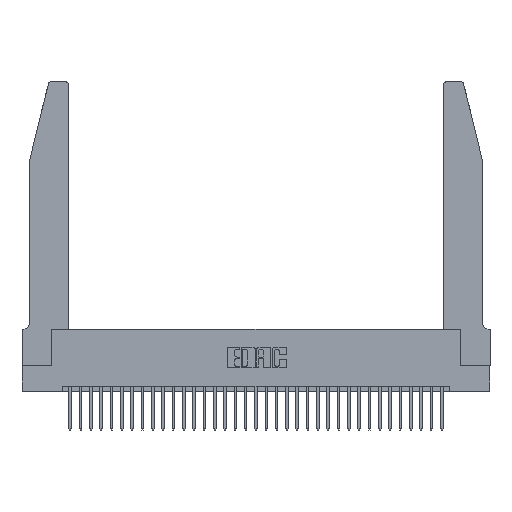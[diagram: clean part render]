
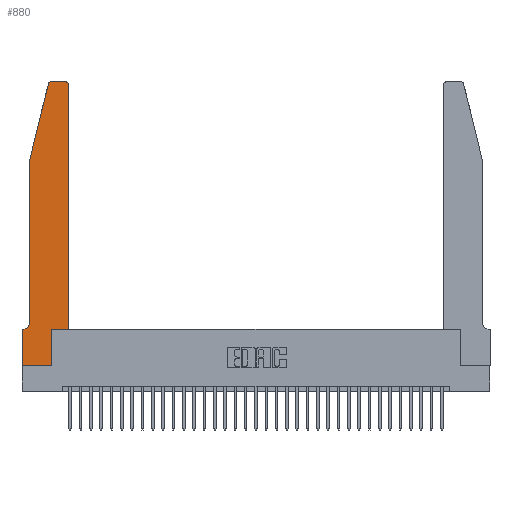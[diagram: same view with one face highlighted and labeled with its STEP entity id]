
A CAD part, top view. The second image highlights one B-rep face of the part: STEP entity #880.
In plain terms, the highlighted planar face has unit normal (0, 0, 1).
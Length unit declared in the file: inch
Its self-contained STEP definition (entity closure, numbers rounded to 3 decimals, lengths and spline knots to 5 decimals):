
#388 = CARTESIAN_POINT ( 'NONE',  ( 0.4505, 0.35, 0.37 ) ) ;
#748 = AXIS2_PLACEMENT_3D ( 'NONE', #17738, #28387, #12498 ) ;
#880 = ADVANCED_FACE ( 'NONE', ( #8861 ), #9839, .T. ) ;
#884 = EDGE_CURVE ( 'NONE', #30929, #30407, #30021, .T. ) ;
#1412 = EDGE_CURVE ( 'NONE', #30407, #5134, #1619, .T. ) ;
#1475 = ORIENTED_EDGE ( 'NONE', *, *, #4021, .T. ) ;
#1619 = CIRCLE ( 'NONE', #23368, 0.03 ) ;
#1680 = CARTESIAN_POINT ( 'NONE',  ( 0.0755, 2., 0.37 ) ) ;
#2343 = ORIENTED_EDGE ( 'NONE', *, *, #17369, .T. ) ;
#2407 = CARTESIAN_POINT ( 'NONE',  ( 0.2865, 0.35, 0.37 ) ) ;
#2535 = VERTEX_POINT ( 'NONE', #22424 ) ;
#2553 = VERTEX_POINT ( 'NONE', #30493 ) ;
#2742 = CARTESIAN_POINT ( 'NONE',  ( 0., 0., 0.37 ) ) ;
#2845 = DIRECTION ( 'NONE',  ( -1., 0., 0. ) ) ;
#2847 = ORIENTED_EDGE ( 'NONE', *, *, #7602, .T. ) ;
#3339 = LINE ( 'NONE', #13101, #30001 ) ;
#3488 = VECTOR ( 'NONE', #2845, 39.37008 ) ;
#4021 = EDGE_CURVE ( 'NONE', #2553, #2535, #23583, .T. ) ;
#4389 = DIRECTION ( 'NONE',  ( 0., 1., 0. ) ) ;
#4568 = LINE ( 'NONE', #26675, #17967 ) ;
#5134 = VERTEX_POINT ( 'NONE', #9296 ) ;
#5929 = AXIS2_PLACEMENT_3D ( 'NONE', #27836, #11956, #30508 ) ;
#6882 = VERTEX_POINT ( 'NONE', #31227 ) ;
#7336 = DIRECTION ( 'NONE',  ( 0., 0., 1. ) ) ;
#7602 = EDGE_CURVE ( 'NONE', #33027, #25494, #3339, .T. ) ;
#8316 = ORIENTED_EDGE ( 'NONE', *, *, #25865, .T. ) ;
#8411 = CARTESIAN_POINT ( 'NONE',  ( 0.2605, 2.75, 0.37 ) ) ;
#8861 = FACE_OUTER_BOUND ( 'NONE', #24070, .T. ) ;
#9197 = VERTEX_POINT ( 'NONE', #29940 ) ;
#9296 = CARTESIAN_POINT ( 'NONE',  ( 0.4205, 2.75, 0.37 ) ) ;
#9839 = PLANE ( 'NONE',  #748 ) ;
#10194 = VERTEX_POINT ( 'NONE', #10356 ) ;
#10215 = CARTESIAN_POINT ( 'NONE',  ( 0.4505, 0.35, 0.37 ) ) ;
#10356 = CARTESIAN_POINT ( 'NONE',  ( 0.25487, 2.72718, 0.37 ) ) ;
#11012 = AXIS2_PLACEMENT_3D ( 'NONE', #27066, #11157, #29722 ) ;
#11157 = DIRECTION ( 'NONE',  ( 0., 0., -1. ) ) ;
#11485 = LINE ( 'NONE', #8411, #3488 ) ;
#11530 = VERTEX_POINT ( 'NONE', #2742 ) ;
#11813 = CARTESIAN_POINT ( 'NONE',  ( 0.0755, 0.35, 0.37 ) ) ;
#11956 = DIRECTION ( 'NONE',  ( 0., 0., 1. ) ) ;
#12245 = LINE ( 'NONE', #20077, #25514 ) ;
#12371 = ORIENTED_EDGE ( 'NONE', *, *, #22803, .T. ) ;
#12498 = DIRECTION ( 'NONE',  ( 1., 0., 0. ) ) ;
#13101 = CARTESIAN_POINT ( 'NONE',  ( 0.2865, 0.35, 0.37 ) ) ;
#13794 = VECTOR ( 'NONE', #32917, 39.37008 ) ;
#14143 = EDGE_CURVE ( 'NONE', #5134, #33887, #11485, .T. ) ;
#14175 = EDGE_CURVE ( 'NONE', #25494, #30929, #24790, .T. ) ;
#14589 = DIRECTION ( 'NONE',  ( -0.239, -0.971, 0. ) ) ;
#14855 = DIRECTION ( 'NONE',  ( 1., 0., 0. ) ) ;
#14951 = EDGE_CURVE ( 'NONE', #33887, #10194, #34245, .T. ) ;
#15005 = EDGE_CURVE ( 'NONE', #11530, #33027, #12245, .T. ) ;
#15693 = ORIENTED_EDGE ( 'NONE', *, *, #14951, .T. ) ;
#15903 = VECTOR ( 'NONE', #4389, 39.37008 ) ;
#16036 = VECTOR ( 'NONE', #32420, 39.37008 ) ;
#17369 = EDGE_CURVE ( 'NONE', #6882, #9197, #27071, .T. ) ;
#17636 = ORIENTED_EDGE ( 'NONE', *, *, #14175, .T. ) ;
#17714 = DIRECTION ( 'NONE',  ( 0., -1., 0. ) ) ;
#17738 = CARTESIAN_POINT ( 'NONE',  ( 0., 0.35, 0.37 ) ) ;
#17967 = VECTOR ( 'NONE', #18784, 39.37008 ) ;
#18201 = VECTOR ( 'NONE', #14589, 39.37008 ) ;
#18783 = ORIENTED_EDGE ( 'NONE', *, *, #15005, .T. ) ;
#18784 = DIRECTION ( 'NONE',  ( 0., -1., 0. ) ) ;
#18838 = CARTESIAN_POINT ( 'NONE',  ( 0.4505, 2.72, 0.37 ) ) ;
#18988 = VECTOR ( 'NONE', #17714, 39.37008 ) ;
#20077 = CARTESIAN_POINT ( 'NONE',  ( 0., 0., 0.37 ) ) ;
#20890 = ORIENTED_EDGE ( 'NONE', *, *, #884, .T. ) ;
#21963 = CARTESIAN_POINT ( 'NONE',  ( 0.284, 2.75, 0.37 ) ) ;
#22424 = CARTESIAN_POINT ( 'NONE',  ( 0.0755, 0.42, 0.37 ) ) ;
#22803 = EDGE_CURVE ( 'NONE', #2535, #6882, #30052, .T. ) ;
#23288 = CARTESIAN_POINT ( 'NONE',  ( 0.4205, 2.72, 0.37 ) ) ;
#23368 = AXIS2_PLACEMENT_3D ( 'NONE', #23288, #7336, #25919 ) ;
#23417 = EDGE_CURVE ( 'NONE', #9197, #11530, #4568, .T. ) ;
#23583 = LINE ( 'NONE', #1680, #18988 ) ;
#23814 = ORIENTED_EDGE ( 'NONE', *, *, #1412, .T. ) ;
#23883 = CARTESIAN_POINT ( 'NONE',  ( 0.2865, 0., 0.37 ) ) ;
#24070 = EDGE_LOOP ( 'NONE', ( #26895, #15693, #8316, #1475, #12371, #2343, #26301, #18783, #2847, #17636, #20890, #23814 ) ) ;
#24790 = LINE ( 'NONE', #388, #16036 ) ;
#25255 = LINE ( 'NONE', #27681, #18201 ) ;
#25494 = VERTEX_POINT ( 'NONE', #2407 ) ;
#25514 = VECTOR ( 'NONE', #14855, 39.37008 ) ;
#25865 = EDGE_CURVE ( 'NONE', #10194, #2553, #25255, .T. ) ;
#25919 = DIRECTION ( 'NONE',  ( 1., 0., 0. ) ) ;
#26301 = ORIENTED_EDGE ( 'NONE', *, *, #23417, .T. ) ;
#26328 = DIRECTION ( 'NONE',  ( 0., 1., 0. ) ) ;
#26675 = CARTESIAN_POINT ( 'NONE',  ( 0., 0., 0.37 ) ) ;
#26895 = ORIENTED_EDGE ( 'NONE', *, *, #14143, .T. ) ;
#27066 = CARTESIAN_POINT ( 'NONE',  ( 0.0055, 0.42, 0.37 ) ) ;
#27071 = LINE ( 'NONE', #11813, #13794 ) ;
#27681 = CARTESIAN_POINT ( 'NONE',  ( 0.0755, 2., 0.37 ) ) ;
#27836 = CARTESIAN_POINT ( 'NONE',  ( 0.284, 2.72, 0.37 ) ) ;
#28387 = DIRECTION ( 'NONE',  ( 0., 0., 1. ) ) ;
#29722 = DIRECTION ( 'NONE',  ( -1., 0., 0. ) ) ;
#29940 = CARTESIAN_POINT ( 'NONE',  ( 0., 0.35, 0.37 ) ) ;
#30001 = VECTOR ( 'NONE', #26328, 39.37008 ) ;
#30021 = LINE ( 'NONE', #31061, #15903 ) ;
#30052 = CIRCLE ( 'NONE', #11012, 0.07 ) ;
#30407 = VERTEX_POINT ( 'NONE', #18838 ) ;
#30493 = CARTESIAN_POINT ( 'NONE',  ( 0.0755, 2., 0.37 ) ) ;
#30508 = DIRECTION ( 'NONE',  ( 1., 0., 0. ) ) ;
#30929 = VERTEX_POINT ( 'NONE', #10215 ) ;
#31061 = CARTESIAN_POINT ( 'NONE',  ( 0.4505, 0.35, 0.37 ) ) ;
#31227 = CARTESIAN_POINT ( 'NONE',  ( 0.0055, 0.35, 0.37 ) ) ;
#32420 = DIRECTION ( 'NONE',  ( 1., 0., 0. ) ) ;
#32917 = DIRECTION ( 'NONE',  ( -1., 0., 0. ) ) ;
#33027 = VERTEX_POINT ( 'NONE', #23883 ) ;
#33887 = VERTEX_POINT ( 'NONE', #21963 ) ;
#34245 = CIRCLE ( 'NONE', #5929, 0.03 ) ;
